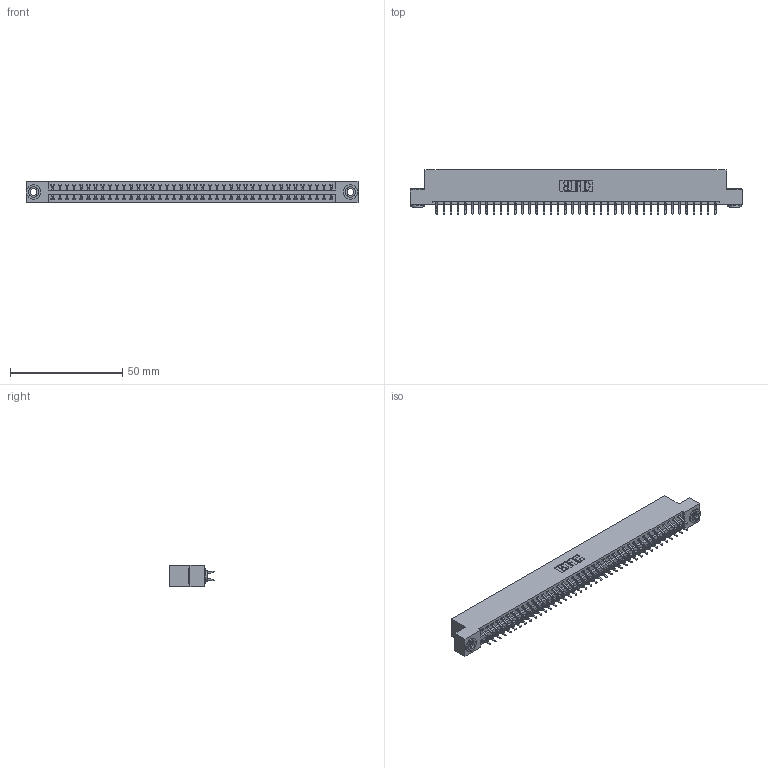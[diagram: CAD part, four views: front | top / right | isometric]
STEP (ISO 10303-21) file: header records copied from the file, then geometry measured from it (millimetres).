
FILE_DESCRIPTION (( 'STEP AP203' ), '1' );
FILE_NAME ('396-080-556-203.STEP', '2018-09-09T21:21:40', ( '' ), ( '' ), 'SwSTEP 2.0', 'SolidWorks 2016', '' );
FILE_SCHEMA (( 'CONFIG_CONTROL_DESIGN' ));
Length unit declared in the file: inch
Products named in the file (4): 396-080-556-203; 346 Part_Flush Mounting Lugs - 0.156 Dia-TH; 345-292-001_556 Tail; 345-250-002_345-250-002-102
Assembly tree (83 placements, depth 2):
  396-080-556-203
    346 Part_Flush Mounting Lugs - 0.156 Dia-TH
    345-292-001_556 Tail  x80
    345-250-002_345-250-002-102  x2
Bounding box: 147.57 x 19.57 x 9.4 mm (x, y, z)
Volume: 14391 mm3; surface area: 19889.8 mm2
Topology: 83 solids, 83 shells, 4800 faces, 14245 edges, 9386 vertices
Faces by surface type: plane 3206, cylinder 1586, cone 8
Entity records: 27244 total; most frequent: CARTESIAN_POINT 4483, ORIENTED_EDGE 4398, DIRECTION 4021, EDGE_CURVE 2199, LINE 1875, VECTOR 1875, VERTEX_POINT 1462, AXIS2_PLACEMENT_3D 1073
